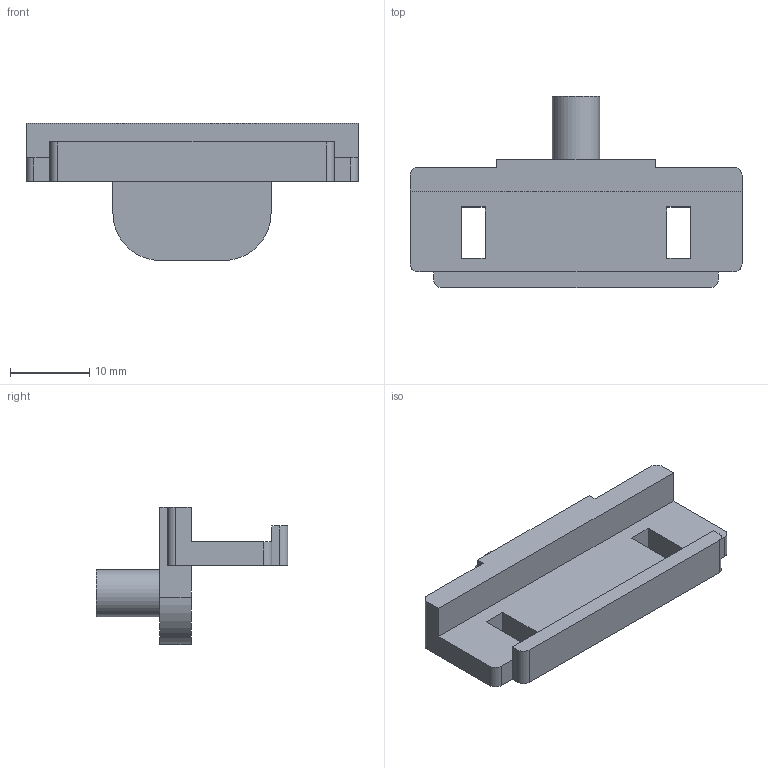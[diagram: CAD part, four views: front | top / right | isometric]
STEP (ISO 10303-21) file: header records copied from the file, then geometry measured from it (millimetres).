
FILE_DESCRIPTION (( 'STEP AP203' ), '1' );
FILE_NAME ('WTF-9_hillbilly_ejector_mount.STEP', '2020-05-09T09:00:52', ( '' ), ( '' ), 'SwSTEP 2.0', 'SolidWorks 2016', '' );
FILE_SCHEMA (( 'CONFIG_CONTROL_DESIGN' ));
Length unit declared in the file: millimetre
Products named in the file (2): WTF-9_hillbilly_ejector_mount; WTF HILLBILLY FINAL_11
Assembly tree (1 placements, depth 2):
  WTF-9_hillbilly_ejector_mount
    WTF HILLBILLY FINAL_11
Bounding box: 42 x 24.2 x 17.34 mm (x, y, z)
Volume: 3558 mm3; surface area: 2793 mm2
Topology: 1 solids, 1 shells, 38 faces, 103 edges, 68 vertices
Faces by surface type: plane 29, cylinder 9
Full cylindrical faces by diameter (mm): 6 x1
Entity records: 1388 total; most frequent: CARTESIAN_POINT 212, ORIENTED_EDGE 204, DIRECTION 204, EDGE_CURVE 102, VECTOR 84, LINE 84, VERTEX_POINT 68, AXIS2_PLACEMENT_3D 60
